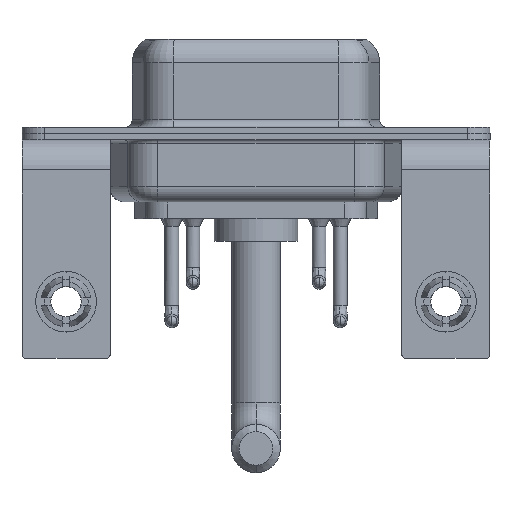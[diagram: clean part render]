
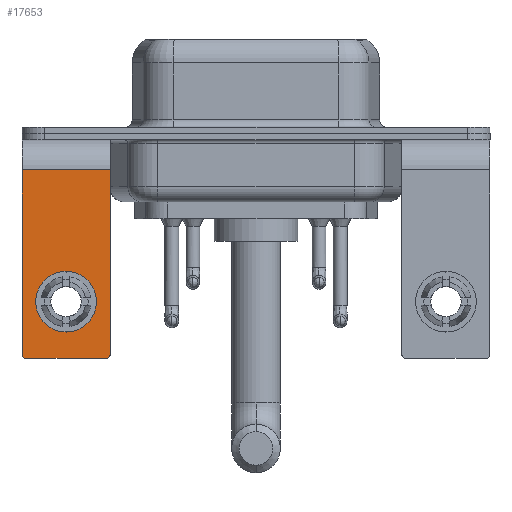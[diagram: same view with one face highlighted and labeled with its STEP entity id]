
A CAD part, front view. The second image highlights one B-rep face of the part: STEP entity #17653.
In plain terms, the highlighted planar face has unit normal (0, -1, 0).
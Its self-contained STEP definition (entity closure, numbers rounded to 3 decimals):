
#640 = LINE ( 'NONE', #17573, #16695 ) ;
#695 = LINE ( 'NONE', #17657, #14396 ) ;
#817 = CIRCLE ( 'NONE', #5047, 0.25 ) ;
#898 = CIRCLE ( 'NONE', #12367, 2. ) ;
#1006 = CARTESIAN_POINT ( 'NONE',  ( 2.9, -6.25, -14.8 ) ) ;
#1159 = DIRECTION ( 'NONE',  ( 0., 0., 1. ) ) ;
#1181 = DIRECTION ( 'NONE',  ( 0., -1., 0. ) ) ;
#1355 = EDGE_CURVE ( 'NONE', #10402, #17602, #4864, .T. ) ;
#1440 = DIRECTION ( 'NONE',  ( 0., 1., 0. ) ) ;
#1606 = ORIENTED_EDGE ( 'NONE', *, *, #5899, .T. ) ;
#1770 = VERTEX_POINT ( 'NONE', #4840 ) ;
#1928 = DIRECTION ( 'NONE',  ( 0., 0., 1. ) ) ;
#2192 = ORIENTED_EDGE ( 'NONE', *, *, #4033, .T. ) ;
#2242 = DIRECTION ( 'NONE',  ( 0., 0., 1. ) ) ;
#2598 = CARTESIAN_POINT ( 'NONE',  ( -2.65, -6.25, -14.55 ) ) ;
#2949 = AXIS2_PLACEMENT_3D ( 'NONE', #4957, #14886, #1928 ) ;
#3539 = EDGE_CURVE ( 'NONE', #10402, #10133, #640, .T. ) ;
#3916 = CARTESIAN_POINT ( 'NONE',  ( 0., -6.25, -11.07 ) ) ;
#4033 = EDGE_CURVE ( 'NONE', #8052, #14018, #817, .T. ) ;
#4267 = EDGE_CURVE ( 'NONE', #1770, #10133, #5365, .T. ) ;
#4347 = ORIENTED_EDGE ( 'NONE', *, *, #7356, .T. ) ;
#4444 = AXIS2_PLACEMENT_3D ( 'NONE', #6607, #12452, #2242 ) ;
#4631 = DIRECTION ( 'NONE',  ( 0., 0., -1. ) ) ;
#4719 = EDGE_CURVE ( 'NONE', #7026, #5910, #898, .T. ) ;
#4840 = CARTESIAN_POINT ( 'NONE',  ( 2.65, -6.25, -14.8 ) ) ;
#4864 = LINE ( 'NONE', #14954, #9429 ) ;
#4957 = CARTESIAN_POINT ( 'NONE',  ( 2.65, -6.25, -14.55 ) ) ;
#5047 = AXIS2_PLACEMENT_3D ( 'NONE', #2598, #1181, #6951 ) ;
#5050 = DIRECTION ( 'NONE',  ( 0., 0., -1. ) ) ;
#5093 = VECTOR ( 'NONE', #9709, 1000. ) ;
#5365 = CIRCLE ( 'NONE', #2949, 0.25 ) ;
#5597 = DIRECTION ( 'NONE',  ( 0., 0., 1. ) ) ;
#5899 = EDGE_CURVE ( 'NONE', #17602, #8052, #695, .T. ) ;
#5910 = VERTEX_POINT ( 'NONE', #13837 ) ;
#6607 = CARTESIAN_POINT ( 'NONE',  ( 2.9, -6.25, -2.4 ) ) ;
#6823 = EDGE_LOOP ( 'NONE', ( #1606, #2192, #14418, #13329, #10919, #8757 ) ) ;
#6951 = DIRECTION ( 'NONE',  ( 0., 0., 1. ) ) ;
#7026 = VERTEX_POINT ( 'NONE', #16483 ) ;
#7176 = CARTESIAN_POINT ( 'NONE',  ( 2.9, -6.25, -14.55 ) ) ;
#7356 = EDGE_CURVE ( 'NONE', #5910, #7026, #17284, .T. ) ;
#7462 = ORIENTED_EDGE ( 'NONE', *, *, #4719, .T. ) ;
#7775 = DIRECTION ( 'NONE',  ( -1., 0., 0. ) ) ;
#7889 = CARTESIAN_POINT ( 'NONE',  ( -2.65, -6.25, -14.8 ) ) ;
#8052 = VERTEX_POINT ( 'NONE', #14423 ) ;
#8757 = ORIENTED_EDGE ( 'NONE', *, *, #1355, .T. ) ;
#8802 = CARTESIAN_POINT ( 'NONE',  ( -2.9, -6.25, -2.4 ) ) ;
#9429 = VECTOR ( 'NONE', #7775, 1000. ) ;
#9709 = DIRECTION ( 'NONE',  ( -1., 0., 0. ) ) ;
#10133 = VERTEX_POINT ( 'NONE', #7176 ) ;
#10402 = VERTEX_POINT ( 'NONE', #13676 ) ;
#10919 = ORIENTED_EDGE ( 'NONE', *, *, #3539, .F. ) ;
#11037 = FACE_BOUND ( 'NONE', #14101, .T. ) ;
#12367 = AXIS2_PLACEMENT_3D ( 'NONE', #3916, #12410, #1159 ) ;
#12410 = DIRECTION ( 'NONE',  ( 0., 1., 0. ) ) ;
#12446 = LINE ( 'NONE', #1006, #5093 ) ;
#12452 = DIRECTION ( 'NONE',  ( 0., 1., 0. ) ) ;
#13329 = ORIENTED_EDGE ( 'NONE', *, *, #4267, .T. ) ;
#13602 = PLANE ( 'NONE',  #4444 ) ;
#13676 = CARTESIAN_POINT ( 'NONE',  ( 2.9, -6.25, -2.4 ) ) ;
#13837 = CARTESIAN_POINT ( 'NONE',  ( 0., -6.25, -13.07 ) ) ;
#13951 = AXIS2_PLACEMENT_3D ( 'NONE', #18559, #1440, #5597 ) ;
#14018 = VERTEX_POINT ( 'NONE', #7889 ) ;
#14101 = EDGE_LOOP ( 'NONE', ( #4347, #7462 ) ) ;
#14396 = VECTOR ( 'NONE', #5050, 1000. ) ;
#14418 = ORIENTED_EDGE ( 'NONE', *, *, #15210, .F. ) ;
#14423 = CARTESIAN_POINT ( 'NONE',  ( -2.9, -6.25, -14.55 ) ) ;
#14886 = DIRECTION ( 'NONE',  ( 0., -1., 0. ) ) ;
#14954 = CARTESIAN_POINT ( 'NONE',  ( 2.9, -6.25, -2.4 ) ) ;
#15210 = EDGE_CURVE ( 'NONE', #1770, #14018, #12446, .T. ) ;
#16483 = CARTESIAN_POINT ( 'NONE',  ( 0., -6.25, -9.07 ) ) ;
#16695 = VECTOR ( 'NONE', #4631, 1000. ) ;
#17284 = CIRCLE ( 'NONE', #13951, 2. ) ;
#17573 = CARTESIAN_POINT ( 'NONE',  ( 2.9, -6.25, -2.4 ) ) ;
#17602 = VERTEX_POINT ( 'NONE', #8802 ) ;
#17653 = ADVANCED_FACE ( 'NONE', ( #11037, #18041 ), #13602, .F. ) ;
#17657 = CARTESIAN_POINT ( 'NONE',  ( -2.9, -6.25, -2.4 ) ) ;
#18041 = FACE_OUTER_BOUND ( 'NONE', #6823, .T. ) ;
#18559 = CARTESIAN_POINT ( 'NONE',  ( 0., -6.25, -11.07 ) ) ;
